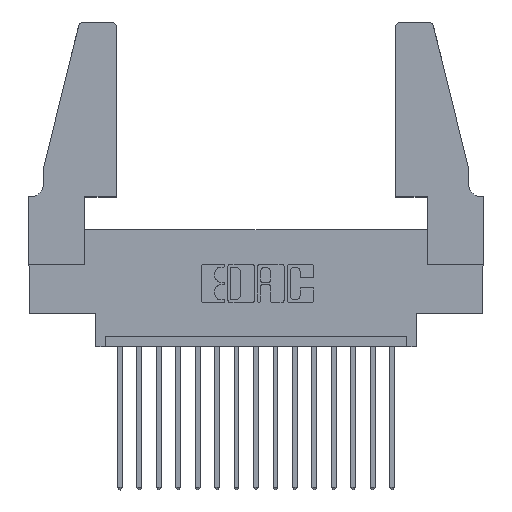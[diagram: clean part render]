
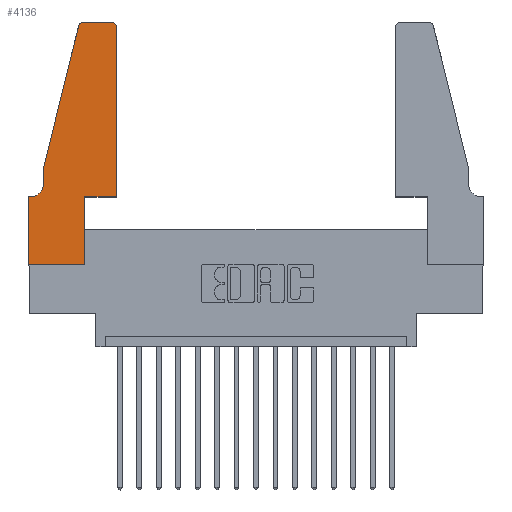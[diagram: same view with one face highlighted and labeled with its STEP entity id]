
A CAD part, top view. The second image highlights one B-rep face of the part: STEP entity #4136.
In plain terms, the highlighted planar face has unit normal (0, 0, 1).
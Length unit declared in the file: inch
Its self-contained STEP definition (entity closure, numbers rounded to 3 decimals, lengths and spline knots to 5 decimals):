
#1 = DIRECTION ( 'NONE',  ( -1., 0., 0. ) ) ;
#162 = EDGE_CURVE ( 'NONE', #9441, #8233, #5552, .T. ) ;
#429 = CARTESIAN_POINT ( 'NONE',  ( 0., 0., 0.37 ) ) ;
#650 = EDGE_CURVE ( 'NONE', #14829, #2755, #9683, .T. ) ;
#756 = AXIS2_PLACEMENT_3D ( 'NONE', #5255, #4216, #14957 ) ;
#795 = CARTESIAN_POINT ( 'NONE',  ( 0.0755, 0.5, 0.37 ) ) ;
#961 = VECTOR ( 'NONE', #16974, 39.37008 ) ;
#1341 = VERTEX_POINT ( 'NONE', #11124 ) ;
#1728 = VERTEX_POINT ( 'NONE', #2575 ) ;
#1874 = CARTESIAN_POINT ( 'NONE',  ( 0.0055, 0.35, 0.37 ) ) ;
#1900 = DIRECTION ( 'NONE',  ( 1., 0., 0. ) ) ;
#1967 = EDGE_CURVE ( 'NONE', #1341, #2543, #16967, .T. ) ;
#2543 = VERTEX_POINT ( 'NONE', #7661 ) ;
#2575 = CARTESIAN_POINT ( 'NONE',  ( 0., 0., 0.37 ) ) ;
#2755 = VERTEX_POINT ( 'NONE', #15701 ) ;
#2884 = EDGE_CURVE ( 'NONE', #17221, #6522, #7114, .T. ) ;
#3140 = AXIS2_PLACEMENT_3D ( 'NONE', #6743, #16072, #14948 ) ;
#3346 = CARTESIAN_POINT ( 'NONE',  ( 0.4205, 1.25, 0.37 ) ) ;
#3495 = LINE ( 'NONE', #795, #17216 ) ;
#3609 = AXIS2_PLACEMENT_3D ( 'NONE', #12452, #7282, #1900 ) ;
#3629 = VECTOR ( 'NONE', #13854, 39.37008 ) ;
#3707 = DIRECTION ( 'NONE',  ( 1., 0., 0. ) ) ;
#3768 = VECTOR ( 'NONE', #3707, 39.37008 ) ;
#3819 = CARTESIAN_POINT ( 'NONE',  ( 0.0755, 0.5, 0.37 ) ) ;
#3833 = VECTOR ( 'NONE', #13165, 39.37008 ) ;
#4074 = CARTESIAN_POINT ( 'NONE',  ( 0., 0.35, 0.37 ) ) ;
#4136 = ADVANCED_FACE ( 'NONE', ( #15227 ), #5310, .T. ) ;
#4141 = DIRECTION ( 'NONE',  ( 0., 0., -1. ) ) ;
#4216 = DIRECTION ( 'NONE',  ( 0., 0., 1. ) ) ;
#4444 = VERTEX_POINT ( 'NONE', #5289 ) ;
#4851 = VECTOR ( 'NONE', #14800, 39.37008 ) ;
#5255 = CARTESIAN_POINT ( 'NONE',  ( 0., 0.35, 0.37 ) ) ;
#5275 = DIRECTION ( 'NONE',  ( 0., 1., 0. ) ) ;
#5289 = CARTESIAN_POINT ( 'NONE',  ( 0.284, 1.25, 0.37 ) ) ;
#5310 = PLANE ( 'NONE',  #756 ) ;
#5472 = DIRECTION ( 'NONE',  ( -1., 0., 0. ) ) ;
#5552 = LINE ( 'NONE', #11695, #961 ) ;
#5613 = CARTESIAN_POINT ( 'NONE',  ( 0.4505, 0.35, 0.37 ) ) ;
#6133 = LINE ( 'NONE', #429, #3629 ) ;
#6251 = LINE ( 'NONE', #6313, #3768 ) ;
#6313 = CARTESIAN_POINT ( 'NONE',  ( 0.4505, 0.35, 0.37 ) ) ;
#6509 = ORIENTED_EDGE ( 'NONE', *, *, #1967, .T. ) ;
#6522 = VERTEX_POINT ( 'NONE', #11265 ) ;
#6743 = CARTESIAN_POINT ( 'NONE',  ( 0.4205, 1.22, 0.37 ) ) ;
#6759 = VERTEX_POINT ( 'NONE', #10957 ) ;
#7114 = LINE ( 'NONE', #14861, #4851 ) ;
#7282 = DIRECTION ( 'NONE',  ( 0., 0., 1. ) ) ;
#7661 = CARTESIAN_POINT ( 'NONE',  ( 0.0755, 0.5, 0.37 ) ) ;
#7905 = LINE ( 'NONE', #13370, #12704 ) ;
#8051 = CIRCLE ( 'NONE', #3140, 0.03 ) ;
#8058 = AXIS2_PLACEMENT_3D ( 'NONE', #12071, #4141, #5472 ) ;
#8233 = VERTEX_POINT ( 'NONE', #4074 ) ;
#8246 = CARTESIAN_POINT ( 'NONE',  ( 0., 0., 0.37 ) ) ;
#8364 = DIRECTION ( 'NONE',  ( 0., -1., 0. ) ) ;
#8581 = ORIENTED_EDGE ( 'NONE', *, *, #8824, .T. ) ;
#8726 = ORIENTED_EDGE ( 'NONE', *, *, #16433, .T. ) ;
#8786 = ORIENTED_EDGE ( 'NONE', *, *, #10131, .T. ) ;
#8824 = EDGE_CURVE ( 'NONE', #8233, #1728, #13063, .T. ) ;
#8848 = ORIENTED_EDGE ( 'NONE', *, *, #2884, .T. ) ;
#9013 = DIRECTION ( 'NONE',  ( 0., -1., 0. ) ) ;
#9122 = ORIENTED_EDGE ( 'NONE', *, *, #162, .T. ) ;
#9304 = EDGE_CURVE ( 'NONE', #2755, #16803, #8051, .T. ) ;
#9441 = VERTEX_POINT ( 'NONE', #1874 ) ;
#9469 = CARTESIAN_POINT ( 'NONE',  ( 0.2865, 0., 0.37 ) ) ;
#9683 = LINE ( 'NONE', #13045, #16371 ) ;
#10131 = EDGE_CURVE ( 'NONE', #4444, #1341, #16180, .T. ) ;
#10295 = EDGE_CURVE ( 'NONE', #2543, #6759, #3495, .T. ) ;
#10328 = ORIENTED_EDGE ( 'NONE', *, *, #14116, .T. ) ;
#10654 = ORIENTED_EDGE ( 'NONE', *, *, #10295, .T. ) ;
#10957 = CARTESIAN_POINT ( 'NONE',  ( 0.0755, 0.42, 0.37 ) ) ;
#11124 = CARTESIAN_POINT ( 'NONE',  ( 0.25487, 1.22718, 0.37 ) ) ;
#11265 = CARTESIAN_POINT ( 'NONE',  ( 0.2865, 0.35, 0.37 ) ) ;
#11695 = CARTESIAN_POINT ( 'NONE',  ( 0.0755, 0.35, 0.37 ) ) ;
#12026 = VECTOR ( 'NONE', #8364, 39.37008 ) ;
#12071 = CARTESIAN_POINT ( 'NONE',  ( 0.0055, 0.42, 0.37 ) ) ;
#12114 = ORIENTED_EDGE ( 'NONE', *, *, #15399, .T. ) ;
#12452 = CARTESIAN_POINT ( 'NONE',  ( 0.284, 1.22, 0.37 ) ) ;
#12704 = VECTOR ( 'NONE', #1, 39.37008 ) ;
#13045 = CARTESIAN_POINT ( 'NONE',  ( 0.4505, 0.35, 0.37 ) ) ;
#13063 = LINE ( 'NONE', #8246, #12026 ) ;
#13165 = DIRECTION ( 'NONE',  ( -0.239, -0.971, 0. ) ) ;
#13370 = CARTESIAN_POINT ( 'NONE',  ( 0.2605, 1.25, 0.37 ) ) ;
#13854 = DIRECTION ( 'NONE',  ( 1., 0., 0. ) ) ;
#14116 = EDGE_CURVE ( 'NONE', #1728, #17221, #6133, .T. ) ;
#14173 = ORIENTED_EDGE ( 'NONE', *, *, #9304, .T. ) ;
#14423 = ORIENTED_EDGE ( 'NONE', *, *, #15355, .T. ) ;
#14800 = DIRECTION ( 'NONE',  ( 0., 1., 0. ) ) ;
#14829 = VERTEX_POINT ( 'NONE', #5613 ) ;
#14836 = ORIENTED_EDGE ( 'NONE', *, *, #650, .T. ) ;
#14861 = CARTESIAN_POINT ( 'NONE',  ( 0.2865, 0.35, 0.37 ) ) ;
#14948 = DIRECTION ( 'NONE',  ( 1., 0., 0. ) ) ;
#14957 = DIRECTION ( 'NONE',  ( 1., 0., 0. ) ) ;
#15227 = FACE_OUTER_BOUND ( 'NONE', #16885, .T. ) ;
#15355 = EDGE_CURVE ( 'NONE', #16803, #4444, #7905, .T. ) ;
#15399 = EDGE_CURVE ( 'NONE', #6759, #9441, #15630, .T. ) ;
#15630 = CIRCLE ( 'NONE', #8058, 0.07 ) ;
#15701 = CARTESIAN_POINT ( 'NONE',  ( 0.4505, 1.22, 0.37 ) ) ;
#16072 = DIRECTION ( 'NONE',  ( 0., 0., 1. ) ) ;
#16180 = CIRCLE ( 'NONE', #3609, 0.03 ) ;
#16371 = VECTOR ( 'NONE', #5275, 39.37008 ) ;
#16433 = EDGE_CURVE ( 'NONE', #6522, #14829, #6251, .T. ) ;
#16803 = VERTEX_POINT ( 'NONE', #3346 ) ;
#16885 = EDGE_LOOP ( 'NONE', ( #14423, #8786, #6509, #10654, #12114, #9122, #8581, #10328, #8848, #8726, #14836, #14173 ) ) ;
#16967 = LINE ( 'NONE', #3819, #3833 ) ;
#16974 = DIRECTION ( 'NONE',  ( -1., 0., 0. ) ) ;
#17216 = VECTOR ( 'NONE', #9013, 39.37008 ) ;
#17221 = VERTEX_POINT ( 'NONE', #9469 ) ;
